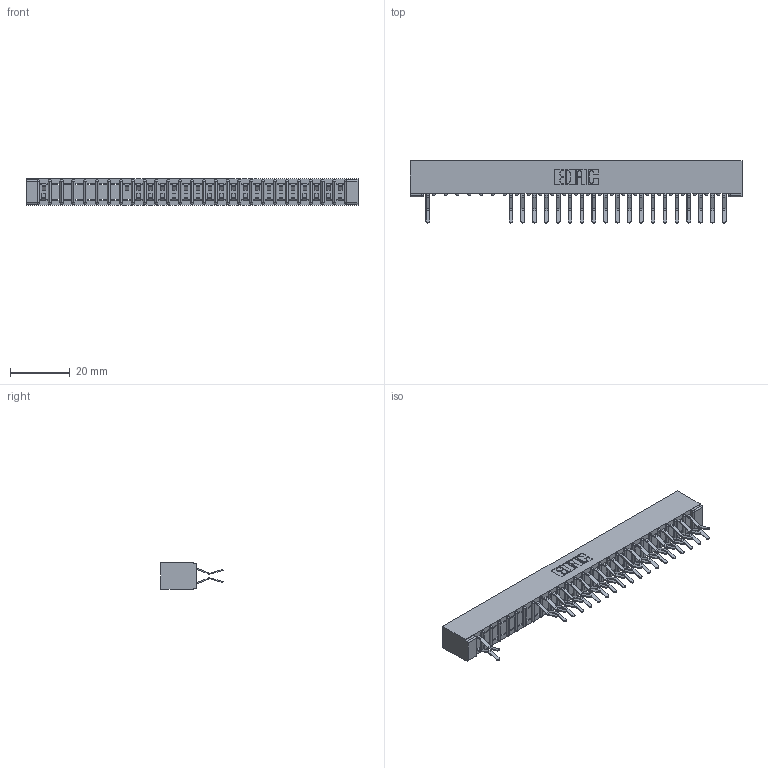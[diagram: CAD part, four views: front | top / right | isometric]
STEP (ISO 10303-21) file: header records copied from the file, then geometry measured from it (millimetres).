
FILE_DESCRIPTION (( 'STEP AP203' ), '1' );
FILE_NAME ('307-052-560-201.STEP', '2018-08-06T05:37:50', ( '' ), ( '' ), 'SwSTEP 2.0', 'SolidWorks 2016', '' );
FILE_SCHEMA (( 'CONFIG_CONTROL_DESIGN' ));
Length unit declared in the file: inch
Products named in the file (3): 307 Part_No Mounting Lugs; 307-290-001_560; 307-052-560-201
Assembly tree (40 placements, depth 2):
  307-052-560-201
    307 Part_No Mounting Lugs
    307-290-001_560  x39
Bounding box: 110.9 x 20.73 x 8.71 mm (x, y, z)
Volume: 7366.8 mm3; surface area: 12992 mm2
Topology: 40 solids, 40 shells, 2217 faces, 6253 edges, 4042 vertices
Faces by surface type: plane 1431, cylinder 732, sphere 54
Entity records: 24504 total; most frequent: CARTESIAN_POINT 4065, ORIENTED_EDGE 4038, DIRECTION 3975, EDGE_CURVE 2019, LINE 1543, VECTOR 1543, VERTEX_POINT 1306, AXIS2_PLACEMENT_3D 1216
